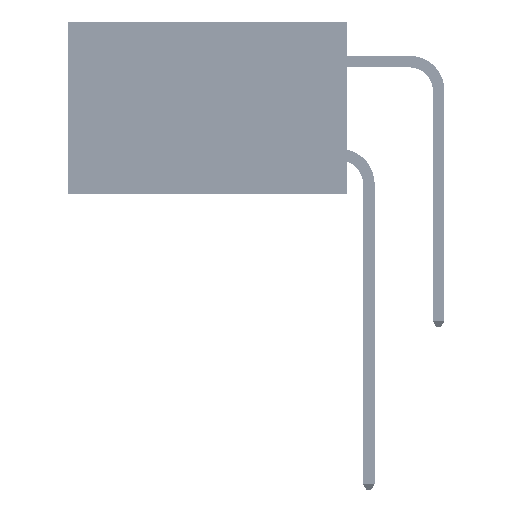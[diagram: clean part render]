
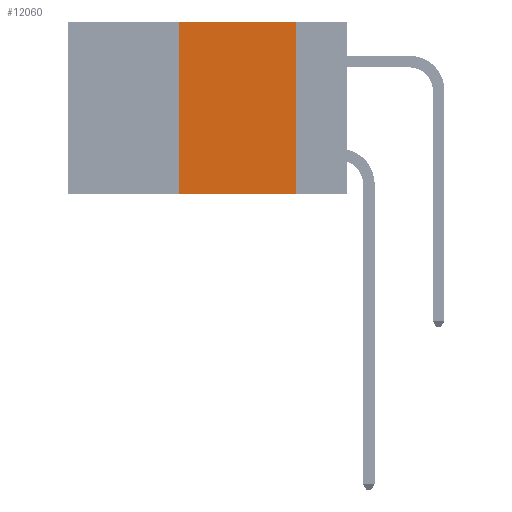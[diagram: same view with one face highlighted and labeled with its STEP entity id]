
A CAD part, left-side view. The second image highlights one B-rep face of the part: STEP entity #12060.
In plain terms, the highlighted planar face has unit normal (-1, 0, 0).
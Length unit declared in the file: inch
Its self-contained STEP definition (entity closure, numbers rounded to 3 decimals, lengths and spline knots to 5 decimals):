
#91 = EDGE_LOOP ( 'NONE', ( #18580, #47119, #19817, #43582 ) ) ;
#193 = DIRECTION ( 'NONE',  ( 0., -1., 0. ) ) ;
#1122 = CARTESIAN_POINT ( 'NONE',  ( 0., 0.11, -0.37 ) ) ;
#1423 = VERTEX_POINT ( 'NONE', #1122 ) ;
#2324 = EDGE_CURVE ( 'NONE', #35251, #1423, #46348, .T. ) ;
#3649 = FACE_OUTER_BOUND ( 'NONE', #91, .T. ) ;
#5535 = EDGE_CURVE ( 'NONE', #8647, #12848, #7517, .T. ) ;
#7517 = LINE ( 'NONE', #47561, #32195 ) ;
#8062 = CARTESIAN_POINT ( 'NONE',  ( 0., 0.36, 0. ) ) ;
#8647 = VERTEX_POINT ( 'NONE', #28333 ) ;
#10497 = PLANE ( 'NONE',  #25766 ) ;
#12060 = ADVANCED_FACE ( 'NONE', ( #3649 ), #10497, .F. ) ;
#12848 = VERTEX_POINT ( 'NONE', #17966 ) ;
#12919 = CARTESIAN_POINT ( 'NONE',  ( 0., 0.6, -0.37 ) ) ;
#16125 = LINE ( 'NONE', #8062, #42086 ) ;
#17966 = CARTESIAN_POINT ( 'NONE',  ( 0., 0.11, 0. ) ) ;
#18580 = ORIENTED_EDGE ( 'NONE', *, *, #23763, .F. ) ;
#19817 = ORIENTED_EDGE ( 'NONE', *, *, #45495, .F. ) ;
#23763 = EDGE_CURVE ( 'NONE', #12848, #1423, #32031, .T. ) ;
#25766 = AXIS2_PLACEMENT_3D ( 'NONE', #32738, #41000, #47590 ) ;
#28333 = CARTESIAN_POINT ( 'NONE',  ( 0., 0.36, 0. ) ) ;
#32031 = LINE ( 'NONE', #35706, #38860 ) ;
#32195 = VECTOR ( 'NONE', #193, 39.37008 ) ;
#32738 = CARTESIAN_POINT ( 'NONE',  ( 0., 0.6, 0. ) ) ;
#35251 = VERTEX_POINT ( 'NONE', #46233 ) ;
#35706 = CARTESIAN_POINT ( 'NONE',  ( 0., 0.11, 0. ) ) ;
#38338 = DIRECTION ( 'NONE',  ( 0., 0., 1. ) ) ;
#38860 = VECTOR ( 'NONE', #42526, 39.37008 ) ;
#41000 = DIRECTION ( 'NONE',  ( 1., 0., 0. ) ) ;
#41944 = DIRECTION ( 'NONE',  ( 0., -1., 0. ) ) ;
#42086 = VECTOR ( 'NONE', #38338, 39.37008 ) ;
#42526 = DIRECTION ( 'NONE',  ( 0., 0., -1. ) ) ;
#42702 = VECTOR ( 'NONE', #41944, 39.37008 ) ;
#43582 = ORIENTED_EDGE ( 'NONE', *, *, #2324, .T. ) ;
#45495 = EDGE_CURVE ( 'NONE', #35251, #8647, #16125, .T. ) ;
#46233 = CARTESIAN_POINT ( 'NONE',  ( 0., 0.36, -0.37 ) ) ;
#46348 = LINE ( 'NONE', #12919, #42702 ) ;
#47119 = ORIENTED_EDGE ( 'NONE', *, *, #5535, .F. ) ;
#47561 = CARTESIAN_POINT ( 'NONE',  ( 0., 0.6, 0. ) ) ;
#47590 = DIRECTION ( 'NONE',  ( 0., 0., -1. ) ) ;
